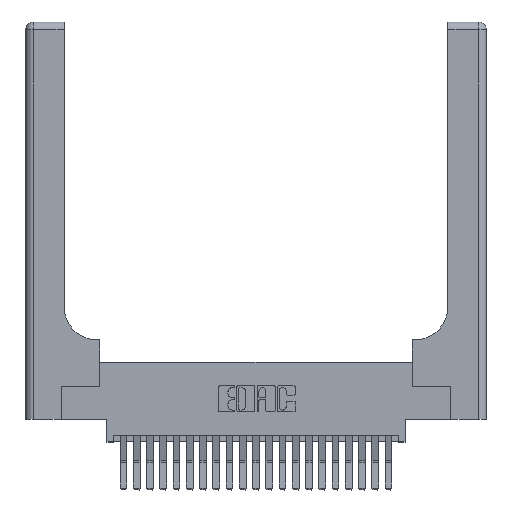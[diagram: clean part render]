
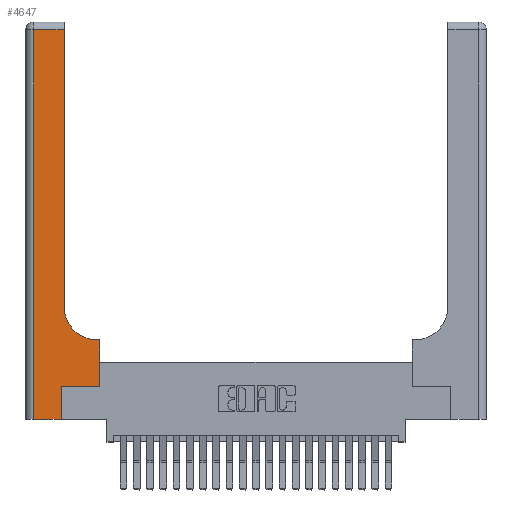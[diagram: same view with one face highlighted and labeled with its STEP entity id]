
A CAD part, top view. The second image highlights one B-rep face of the part: STEP entity #4647.
In plain terms, the highlighted planar face has unit normal (0, 0, 1).
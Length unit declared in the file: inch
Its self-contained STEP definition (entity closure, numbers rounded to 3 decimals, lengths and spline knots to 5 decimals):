
#483 = CIRCLE ( 'NONE', #8019, 0.25 ) ;
#507 = VERTEX_POINT ( 'NONE', #10614 ) ;
#1051 = DIRECTION ( 'NONE',  ( 0., 1., 0. ) ) ;
#1726 = VERTEX_POINT ( 'NONE', #8058 ) ;
#1940 = DIRECTION ( 'NONE',  ( -1., 0., 0. ) ) ;
#2000 = VERTEX_POINT ( 'NONE', #3240 ) ;
#2059 = VECTOR ( 'NONE', #1051, 39.37008 ) ;
#2566 = CARTESIAN_POINT ( 'NONE',  ( 0.5415, 0.85, 0.37 ) ) ;
#2567 = VERTEX_POINT ( 'NONE', #20337 ) ;
#2963 = LINE ( 'NONE', #24715, #12501 ) ;
#3086 = EDGE_CURVE ( 'NONE', #8005, #1726, #10035, .T. ) ;
#3240 = CARTESIAN_POINT ( 'NONE',  ( 0.06, 2.94, 0.37 ) ) ;
#3365 = EDGE_CURVE ( 'NONE', #2000, #17766, #23764, .T. ) ;
#3443 = VECTOR ( 'NONE', #22017, 39.37008 ) ;
#3830 = DIRECTION ( 'NONE',  ( 0., 1., 0. ) ) ;
#4494 = DIRECTION ( 'NONE',  ( 1., 0., 0. ) ) ;
#4647 = ADVANCED_FACE ( 'NONE', ( #18291 ), #17138, .F. ) ;
#4855 = VERTEX_POINT ( 'NONE', #4997 ) ;
#4997 = CARTESIAN_POINT ( 'NONE',  ( 0.2915, 0.85, 0.37 ) ) ;
#5059 = EDGE_CURVE ( 'NONE', #4855, #507, #18273, .T. ) ;
#5627 = ORIENTED_EDGE ( 'NONE', *, *, #5059, .T. ) ;
#5695 = CARTESIAN_POINT ( 'NONE',  ( 0., 2.94, 0.37 ) ) ;
#6782 = EDGE_CURVE ( 'NONE', #9378, #8005, #2963, .T. ) ;
#6893 = CARTESIAN_POINT ( 'NONE',  ( 0.269, 0.25, 0.37 ) ) ;
#7117 = LINE ( 'NONE', #20103, #2059 ) ;
#7559 = DIRECTION ( 'NONE',  ( -1., 0., 0. ) ) ;
#7612 = ORIENTED_EDGE ( 'NONE', *, *, #20652, .T. ) ;
#7653 = CARTESIAN_POINT ( 'NONE',  ( 0.06, 3., 0.37 ) ) ;
#7850 = DIRECTION ( 'NONE',  ( 1., 0., 0. ) ) ;
#8005 = VERTEX_POINT ( 'NONE', #17596 ) ;
#8019 = AXIS2_PLACEMENT_3D ( 'NONE', #2566, #15952, #4494 ) ;
#8058 = CARTESIAN_POINT ( 'NONE',  ( 0.5585, 0.25, 0.37 ) ) ;
#8063 = VECTOR ( 'NONE', #3830, 39.37008 ) ;
#8205 = VECTOR ( 'NONE', #7850, 39.37008 ) ;
#8473 = LINE ( 'NONE', #19998, #3443 ) ;
#9115 = ORIENTED_EDGE ( 'NONE', *, *, #3086, .T. ) ;
#9378 = VERTEX_POINT ( 'NONE', #19162 ) ;
#9439 = VECTOR ( 'NONE', #22235, 39.37008 ) ;
#9973 = VERTEX_POINT ( 'NONE', #11674 ) ;
#10035 = LINE ( 'NONE', #6893, #9439 ) ;
#10614 = CARTESIAN_POINT ( 'NONE',  ( 0.2915, 2.94, 0.37 ) ) ;
#11011 = CARTESIAN_POINT ( 'NONE',  ( 0.06, 0., 0.37 ) ) ;
#11259 = DIRECTION ( 'NONE',  ( 0., 1., 0. ) ) ;
#11674 = CARTESIAN_POINT ( 'NONE',  ( 0.5415, 0.6, 0.37 ) ) ;
#12501 = VECTOR ( 'NONE', #11259, 39.37008 ) ;
#13320 = LINE ( 'NONE', #21260, #8205 ) ;
#13457 = EDGE_LOOP ( 'NONE', ( #5627, #15956, #18754, #21324, #14755, #9115, #7612, #20605, #23022 ) ) ;
#14755 = ORIENTED_EDGE ( 'NONE', *, *, #6782, .T. ) ;
#15952 = DIRECTION ( 'NONE',  ( 0., 0., -1. ) ) ;
#15956 = ORIENTED_EDGE ( 'NONE', *, *, #21586, .T. ) ;
#17138 = PLANE ( 'NONE',  #23952 ) ;
#17301 = VECTOR ( 'NONE', #1940, 39.37008 ) ;
#17596 = CARTESIAN_POINT ( 'NONE',  ( 0.269, 0.25, 0.37 ) ) ;
#17766 = VERTEX_POINT ( 'NONE', #11011 ) ;
#18273 = LINE ( 'NONE', #19111, #8063 ) ;
#18291 = FACE_OUTER_BOUND ( 'NONE', #13457, .T. ) ;
#18715 = VECTOR ( 'NONE', #21051, 39.37008 ) ;
#18754 = ORIENTED_EDGE ( 'NONE', *, *, #3365, .T. ) ;
#19051 = DIRECTION ( 'NONE',  ( 0., 0., -1. ) ) ;
#19111 = CARTESIAN_POINT ( 'NONE',  ( 0.2915, 3., 0.37 ) ) ;
#19162 = CARTESIAN_POINT ( 'NONE',  ( 0.269, 0., 0.37 ) ) ;
#19998 = CARTESIAN_POINT ( 'NONE',  ( 0.2915, 0.6, 0.37 ) ) ;
#20103 = CARTESIAN_POINT ( 'NONE',  ( 0.5585, 0.25, 0.37 ) ) ;
#20337 = CARTESIAN_POINT ( 'NONE',  ( 0.5585, 0.6, 0.37 ) ) ;
#20605 = ORIENTED_EDGE ( 'NONE', *, *, #23191, .T. ) ;
#20652 = EDGE_CURVE ( 'NONE', #1726, #2567, #7117, .T. ) ;
#21051 = DIRECTION ( 'NONE',  ( 0., -1., 0. ) ) ;
#21260 = CARTESIAN_POINT ( 'NONE',  ( 0., 0., 0.37 ) ) ;
#21324 = ORIENTED_EDGE ( 'NONE', *, *, #23595, .T. ) ;
#21586 = EDGE_CURVE ( 'NONE', #507, #2000, #22958, .T. ) ;
#22017 = DIRECTION ( 'NONE',  ( -1., 0., 0. ) ) ;
#22235 = DIRECTION ( 'NONE',  ( 1., 0., 0. ) ) ;
#22394 = EDGE_CURVE ( 'NONE', #9973, #4855, #483, .T. ) ;
#22958 = LINE ( 'NONE', #5695, #17301 ) ;
#23022 = ORIENTED_EDGE ( 'NONE', *, *, #22394, .T. ) ;
#23191 = EDGE_CURVE ( 'NONE', #2567, #9973, #8473, .T. ) ;
#23595 = EDGE_CURVE ( 'NONE', #17766, #9378, #13320, .T. ) ;
#23764 = LINE ( 'NONE', #7653, #18715 ) ;
#23952 = AXIS2_PLACEMENT_3D ( 'NONE', #24704, #19051, #7559 ) ;
#24704 = CARTESIAN_POINT ( 'NONE',  ( 0., 3., 0.37 ) ) ;
#24715 = CARTESIAN_POINT ( 'NONE',  ( 0.269, 0., 0.37 ) ) ;
